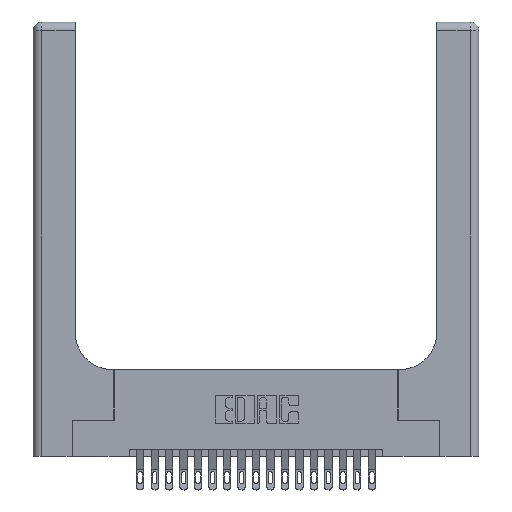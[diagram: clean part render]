
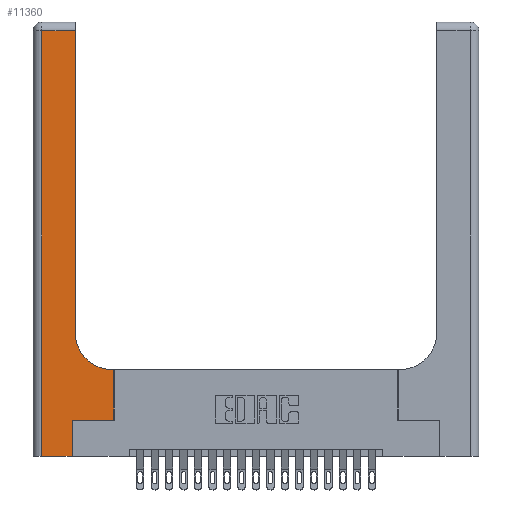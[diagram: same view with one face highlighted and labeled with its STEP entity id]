
A CAD part, top view. The second image highlights one B-rep face of the part: STEP entity #11360.
In plain terms, the highlighted planar face has unit normal (0, 0, 1).
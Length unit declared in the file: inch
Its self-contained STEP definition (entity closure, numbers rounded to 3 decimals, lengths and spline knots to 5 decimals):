
#48 = CARTESIAN_POINT ( 'NONE',  ( 0.2915, 3., 0.37 ) ) ;
#49 = CARTESIAN_POINT ( 'NONE',  ( 0.06, 3., 0.37 ) ) ;
#363 = VECTOR ( 'NONE', #12362, 39.37008 ) ;
#499 = CIRCLE ( 'NONE', #19612, 0.25 ) ;
#677 = LINE ( 'NONE', #13750, #4757 ) ;
#1029 = VECTOR ( 'NONE', #19793, 39.37008 ) ;
#1121 = EDGE_CURVE ( 'NONE', #4675, #4417, #6171, .T. ) ;
#1556 = VERTEX_POINT ( 'NONE', #20744 ) ;
#2027 = DIRECTION ( 'NONE',  ( 0., 1., 0. ) ) ;
#3447 = DIRECTION ( 'NONE',  ( -1., 0., 0. ) ) ;
#3503 = DIRECTION ( 'NONE',  ( 0., 1., 0. ) ) ;
#4417 = VERTEX_POINT ( 'NONE', #7683 ) ;
#4675 = VERTEX_POINT ( 'NONE', #21895 ) ;
#4757 = VECTOR ( 'NONE', #3447, 39.37008 ) ;
#5001 = LINE ( 'NONE', #10672, #363 ) ;
#5411 = LINE ( 'NONE', #48, #18602 ) ;
#5482 = VECTOR ( 'NONE', #21419, 39.37008 ) ;
#5704 = VERTEX_POINT ( 'NONE', #17792 ) ;
#6032 = PLANE ( 'NONE',  #7292 ) ;
#6090 = CARTESIAN_POINT ( 'NONE',  ( 0.2915, 0.85, 0.37 ) ) ;
#6171 = LINE ( 'NONE', #12857, #14260 ) ;
#6516 = EDGE_CURVE ( 'NONE', #4417, #13236, #499, .T. ) ;
#6533 = DIRECTION ( 'NONE',  ( 0., 0., -1. ) ) ;
#6943 = EDGE_CURVE ( 'NONE', #19428, #21139, #14267, .T. ) ;
#7292 = AXIS2_PLACEMENT_3D ( 'NONE', #18079, #7797, #19772 ) ;
#7683 = CARTESIAN_POINT ( 'NONE',  ( 0.5415, 0.6, 0.37 ) ) ;
#7742 = CARTESIAN_POINT ( 'NONE',  ( 0.269, 0.25, 0.37 ) ) ;
#7776 = CARTESIAN_POINT ( 'NONE',  ( 0.269, 0., 0.37 ) ) ;
#7797 = DIRECTION ( 'NONE',  ( 0., 0., -1. ) ) ;
#7818 = CARTESIAN_POINT ( 'NONE',  ( 0.269, 0.25, 0.37 ) ) ;
#8193 = VERTEX_POINT ( 'NONE', #14907 ) ;
#8593 = FACE_OUTER_BOUND ( 'NONE', #8745, .T. ) ;
#8745 = EDGE_LOOP ( 'NONE', ( #14534, #14447, #14356, #15151, #15060, #15113, #15278, #14860, #14922 ) ) ;
#9181 = EDGE_CURVE ( 'NONE', #13236, #8193, #5411, .T. ) ;
#10115 = LINE ( 'NONE', #7776, #5482 ) ;
#10169 = VERTEX_POINT ( 'NONE', #17616 ) ;
#10477 = DIRECTION ( 'NONE',  ( 0., -1., 0. ) ) ;
#10672 = CARTESIAN_POINT ( 'NONE',  ( 0., 0., 0.37 ) ) ;
#10806 = CARTESIAN_POINT ( 'NONE',  ( 0.5585, 0.25, 0.37 ) ) ;
#11160 = EDGE_CURVE ( 'NONE', #1556, #5704, #21878, .T. ) ;
#11360 = ADVANCED_FACE ( 'NONE', ( #8593 ), #6032, .F. ) ;
#12299 = EDGE_CURVE ( 'NONE', #8193, #1556, #677, .T. ) ;
#12362 = DIRECTION ( 'NONE',  ( 1., 0., 0. ) ) ;
#12857 = CARTESIAN_POINT ( 'NONE',  ( 0.2915, 0.6, 0.37 ) ) ;
#12954 = EDGE_CURVE ( 'NONE', #5704, #10169, #5001, .T. ) ;
#13236 = VERTEX_POINT ( 'NONE', #6090 ) ;
#13750 = CARTESIAN_POINT ( 'NONE',  ( 0., 2.94, 0.37 ) ) ;
#14260 = VECTOR ( 'NONE', #16342, 39.37008 ) ;
#14267 = LINE ( 'NONE', #7818, #1029 ) ;
#14356 = ORIENTED_EDGE ( 'NONE', *, *, #11160, .T. ) ;
#14447 = ORIENTED_EDGE ( 'NONE', *, *, #12299, .T. ) ;
#14534 = ORIENTED_EDGE ( 'NONE', *, *, #9181, .T. ) ;
#14860 = ORIENTED_EDGE ( 'NONE', *, *, #1121, .T. ) ;
#14907 = CARTESIAN_POINT ( 'NONE',  ( 0.2915, 2.94, 0.37 ) ) ;
#14922 = ORIENTED_EDGE ( 'NONE', *, *, #6516, .T. ) ;
#15060 = ORIENTED_EDGE ( 'NONE', *, *, #20520, .T. ) ;
#15113 = ORIENTED_EDGE ( 'NONE', *, *, #6943, .T. ) ;
#15151 = ORIENTED_EDGE ( 'NONE', *, *, #12954, .T. ) ;
#15278 = ORIENTED_EDGE ( 'NONE', *, *, #18565, .T. ) ;
#16342 = DIRECTION ( 'NONE',  ( -1., 0., 0. ) ) ;
#16856 = CARTESIAN_POINT ( 'NONE',  ( 0.5415, 0.85, 0.37 ) ) ;
#16910 = VECTOR ( 'NONE', #10477, 39.37008 ) ;
#17143 = VECTOR ( 'NONE', #2027, 39.37008 ) ;
#17552 = CARTESIAN_POINT ( 'NONE',  ( 0.5585, 0.25, 0.37 ) ) ;
#17616 = CARTESIAN_POINT ( 'NONE',  ( 0.269, 0., 0.37 ) ) ;
#17792 = CARTESIAN_POINT ( 'NONE',  ( 0.06, 0., 0.37 ) ) ;
#18079 = CARTESIAN_POINT ( 'NONE',  ( 0., 3., 0.37 ) ) ;
#18565 = EDGE_CURVE ( 'NONE', #21139, #4675, #21070, .T. ) ;
#18578 = DIRECTION ( 'NONE',  ( 1., 0., 0. ) ) ;
#18602 = VECTOR ( 'NONE', #3503, 39.37008 ) ;
#19428 = VERTEX_POINT ( 'NONE', #7742 ) ;
#19612 = AXIS2_PLACEMENT_3D ( 'NONE', #16856, #6533, #18578 ) ;
#19772 = DIRECTION ( 'NONE',  ( -1., 0., 0. ) ) ;
#19793 = DIRECTION ( 'NONE',  ( 1., 0., 0. ) ) ;
#20520 = EDGE_CURVE ( 'NONE', #10169, #19428, #10115, .T. ) ;
#20744 = CARTESIAN_POINT ( 'NONE',  ( 0.06, 2.94, 0.37 ) ) ;
#21070 = LINE ( 'NONE', #17552, #17143 ) ;
#21139 = VERTEX_POINT ( 'NONE', #10806 ) ;
#21419 = DIRECTION ( 'NONE',  ( 0., 1., 0. ) ) ;
#21878 = LINE ( 'NONE', #49, #16910 ) ;
#21895 = CARTESIAN_POINT ( 'NONE',  ( 0.5585, 0.6, 0.37 ) ) ;
